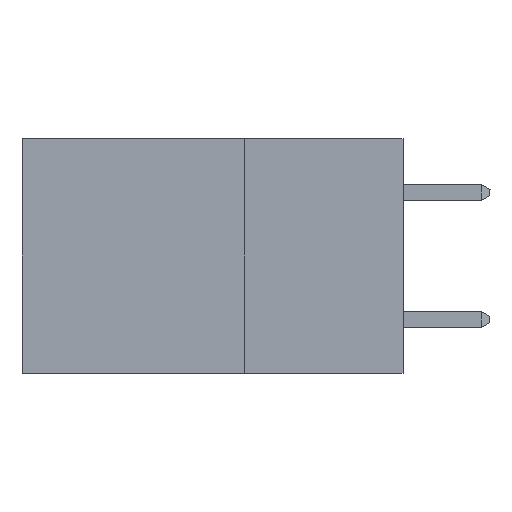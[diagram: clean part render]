
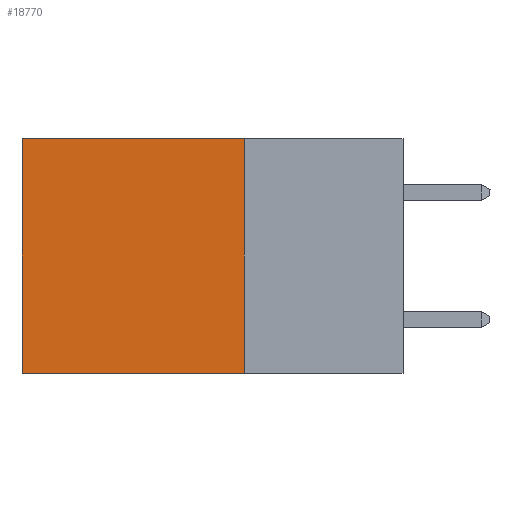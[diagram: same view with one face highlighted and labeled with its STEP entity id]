
A CAD part, left-side view. The second image highlights one B-rep face of the part: STEP entity #18770.
In plain terms, the highlighted planar face has unit normal (-1, 0, 0).
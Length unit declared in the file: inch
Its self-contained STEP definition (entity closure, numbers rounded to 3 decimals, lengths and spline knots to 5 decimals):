
#49 = VERTEX_POINT ( 'NONE', #9744 ) ;
#205 = CARTESIAN_POINT ( 'NONE',  ( 0.2875, 0.25, 0. ) ) ;
#1236 = VECTOR ( 'NONE', #24027, 39.37008 ) ;
#1238 = VECTOR ( 'NONE', #8040, 39.37008 ) ;
#1877 = LINE ( 'NONE', #205, #1238 ) ;
#2108 = DIRECTION ( 'NONE',  ( 1., 0., 0. ) ) ;
#2858 = ORIENTED_EDGE ( 'NONE', *, *, #4848, .T. ) ;
#3623 = CARTESIAN_POINT ( 'NONE',  ( 0.2875, 0.25, -0.37 ) ) ;
#4848 = EDGE_CURVE ( 'NONE', #20505, #19681, #22434, .T. ) ;
#7184 = VECTOR ( 'NONE', #7192, 39.37008 ) ;
#7192 = DIRECTION ( 'NONE',  ( 0., 1., 0. ) ) ;
#7546 = AXIS2_PLACEMENT_3D ( 'NONE', #9826, #2108, #7967 ) ;
#7884 = VERTEX_POINT ( 'NONE', #3623 ) ;
#7967 = DIRECTION ( 'NONE',  ( 0., 0., -1. ) ) ;
#8040 = DIRECTION ( 'NONE',  ( 0., 0., -1. ) ) ;
#8352 = CARTESIAN_POINT ( 'NONE',  ( 0.2875, 0.6, 0. ) ) ;
#9224 = VECTOR ( 'NONE', #20556, 39.37008 ) ;
#9343 = CARTESIAN_POINT ( 'NONE',  ( 0.2875, 0.25, 0. ) ) ;
#9744 = CARTESIAN_POINT ( 'NONE',  ( 0.2875, 0.6, -0.37 ) ) ;
#9826 = CARTESIAN_POINT ( 'NONE',  ( 0.2875, 0.25, 0. ) ) ;
#10019 = EDGE_LOOP ( 'NONE', ( #11869, #20052, #16322, #2858 ) ) ;
#11209 = CARTESIAN_POINT ( 'NONE',  ( 0.2875, 0.25, -0.37 ) ) ;
#11869 = ORIENTED_EDGE ( 'NONE', *, *, #12077, .T. ) ;
#12077 = EDGE_CURVE ( 'NONE', #19681, #49, #24378, .T. ) ;
#13010 = CARTESIAN_POINT ( 'NONE',  ( 0.2875, 0.6, 0. ) ) ;
#14265 = CARTESIAN_POINT ( 'NONE',  ( 0.2875, 0.25, 0. ) ) ;
#16322 = ORIENTED_EDGE ( 'NONE', *, *, #18096, .F. ) ;
#17294 = PLANE ( 'NONE',  #7546 ) ;
#17416 = EDGE_CURVE ( 'NONE', #7884, #49, #19833, .T. ) ;
#18096 = EDGE_CURVE ( 'NONE', #20505, #7884, #1877, .T. ) ;
#18770 = ADVANCED_FACE ( 'NONE', ( #19094 ), #17294, .F. ) ;
#19094 = FACE_OUTER_BOUND ( 'NONE', #10019, .T. ) ;
#19681 = VERTEX_POINT ( 'NONE', #8352 ) ;
#19833 = LINE ( 'NONE', #11209, #7184 ) ;
#20052 = ORIENTED_EDGE ( 'NONE', *, *, #17416, .F. ) ;
#20505 = VERTEX_POINT ( 'NONE', #9343 ) ;
#20556 = DIRECTION ( 'NONE',  ( 0., 0., -1. ) ) ;
#22434 = LINE ( 'NONE', #14265, #1236 ) ;
#24027 = DIRECTION ( 'NONE',  ( 0., 1., 0. ) ) ;
#24378 = LINE ( 'NONE', #13010, #9224 ) ;
